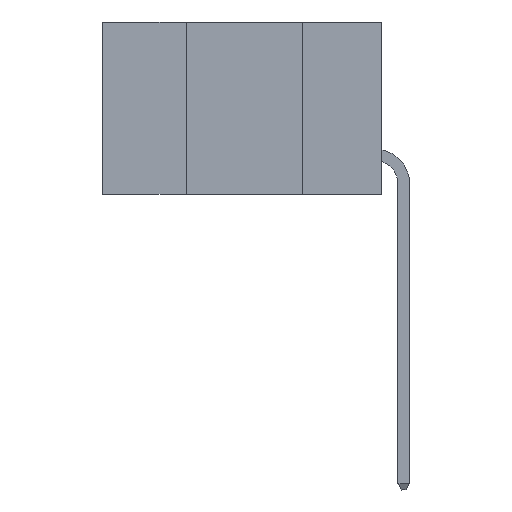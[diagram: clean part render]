
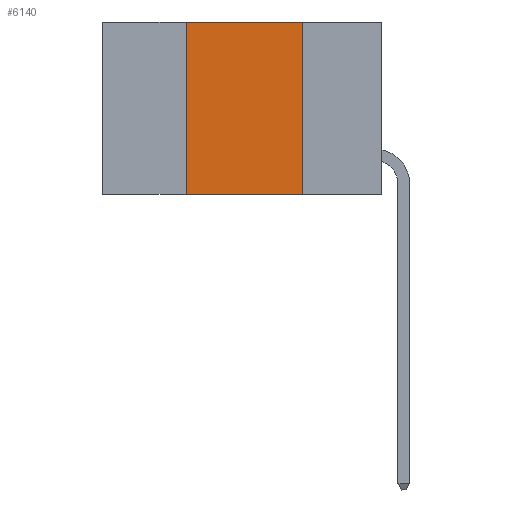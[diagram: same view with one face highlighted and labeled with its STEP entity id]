
A CAD part, left-side view. The second image highlights one B-rep face of the part: STEP entity #6140.
In plain terms, the highlighted planar face has unit normal (-1, 0, 0).
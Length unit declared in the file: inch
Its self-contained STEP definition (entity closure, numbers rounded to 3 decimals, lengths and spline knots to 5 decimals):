
#165 = VECTOR ( 'NONE', #10172, 39.37008 ) ;
#1173 = FACE_OUTER_BOUND ( 'NONE', #8826, .T. ) ;
#1730 = DIRECTION ( 'NONE',  ( 1., 0., 0. ) ) ;
#2863 = VECTOR ( 'NONE', #6031, 39.37008 ) ;
#2927 = VERTEX_POINT ( 'NONE', #9703 ) ;
#3143 = ORIENTED_EDGE ( 'NONE', *, *, #4665, .T. ) ;
#3526 = CARTESIAN_POINT ( 'NONE',  ( 0., 0.42, -0.37 ) ) ;
#3738 = VERTEX_POINT ( 'NONE', #5189 ) ;
#3898 = CARTESIAN_POINT ( 'NONE',  ( 0., 0.6, 0. ) ) ;
#4665 = EDGE_CURVE ( 'NONE', #8796, #3738, #5439, .T. ) ;
#5087 = LINE ( 'NONE', #7089, #9604 ) ;
#5189 = CARTESIAN_POINT ( 'NONE',  ( 0., 0.17, -0.37 ) ) ;
#5439 = LINE ( 'NONE', #9569, #2863 ) ;
#5548 = LINE ( 'NONE', #6683, #165 ) ;
#5817 = DIRECTION ( 'NONE',  ( 0., -1., 0. ) ) ;
#6031 = DIRECTION ( 'NONE',  ( 0., -1., 0. ) ) ;
#6140 = ADVANCED_FACE ( 'NONE', ( #1173 ), #9248, .F. ) ;
#6173 = EDGE_CURVE ( 'NONE', #2927, #3738, #5548, .T. ) ;
#6683 = CARTESIAN_POINT ( 'NONE',  ( 0., 0.17, 0. ) ) ;
#7089 = CARTESIAN_POINT ( 'NONE',  ( 0., 0.42, 0. ) ) ;
#7167 = VECTOR ( 'NONE', #5817, 39.37008 ) ;
#7980 = DIRECTION ( 'NONE',  ( 0., 0., 1. ) ) ;
#8140 = VERTEX_POINT ( 'NONE', #11343 ) ;
#8403 = DIRECTION ( 'NONE',  ( 0., 0., -1. ) ) ;
#8796 = VERTEX_POINT ( 'NONE', #3526 ) ;
#8826 = EDGE_LOOP ( 'NONE', ( #9874, #12024, #10123, #3143 ) ) ;
#8919 = AXIS2_PLACEMENT_3D ( 'NONE', #10912, #1730, #8403 ) ;
#9248 = PLANE ( 'NONE',  #8919 ) ;
#9510 = LINE ( 'NONE', #3898, #7167 ) ;
#9569 = CARTESIAN_POINT ( 'NONE',  ( 0., 0.6, -0.37 ) ) ;
#9604 = VECTOR ( 'NONE', #7980, 39.37008 ) ;
#9703 = CARTESIAN_POINT ( 'NONE',  ( 0., 0.17, 0. ) ) ;
#9846 = EDGE_CURVE ( 'NONE', #8140, #2927, #9510, .T. ) ;
#9874 = ORIENTED_EDGE ( 'NONE', *, *, #6173, .F. ) ;
#10123 = ORIENTED_EDGE ( 'NONE', *, *, #11369, .F. ) ;
#10172 = DIRECTION ( 'NONE',  ( 0., 0., -1. ) ) ;
#10912 = CARTESIAN_POINT ( 'NONE',  ( 0., 0.6, 0. ) ) ;
#11343 = CARTESIAN_POINT ( 'NONE',  ( 0., 0.42, 0. ) ) ;
#11369 = EDGE_CURVE ( 'NONE', #8796, #8140, #5087, .T. ) ;
#12024 = ORIENTED_EDGE ( 'NONE', *, *, #9846, .F. ) ;
